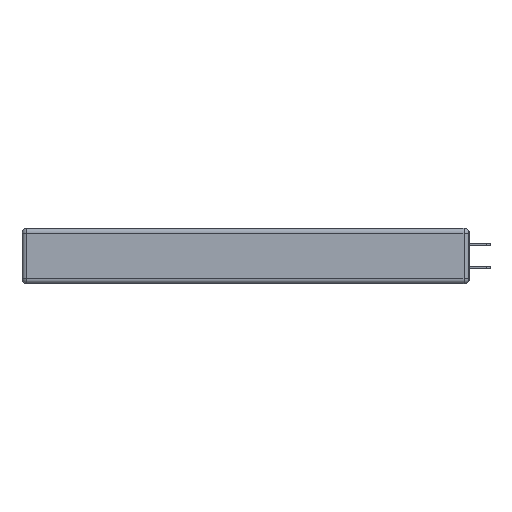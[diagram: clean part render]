
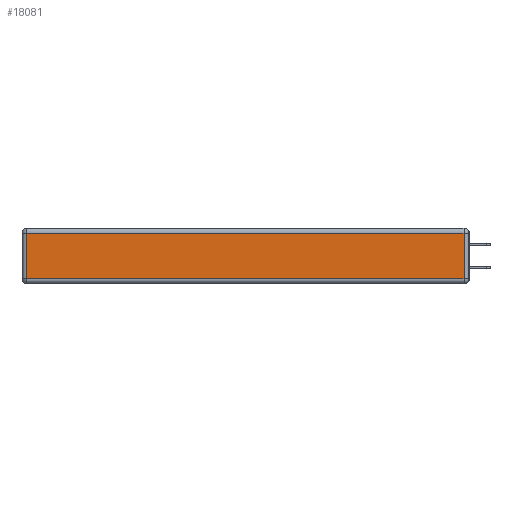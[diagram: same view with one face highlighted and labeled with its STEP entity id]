
A CAD part, left-side view. The second image highlights one B-rep face of the part: STEP entity #18081.
In plain terms, the highlighted planar face has unit normal (-1, 0, 0).
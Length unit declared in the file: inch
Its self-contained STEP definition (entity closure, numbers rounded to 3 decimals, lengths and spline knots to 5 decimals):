
#25 = VECTOR ( 'NONE', #11373, 39.37008 ) ;
#868 = DIRECTION ( 'NONE',  ( 0., 0., 1. ) ) ;
#2561 = VECTOR ( 'NONE', #9159, 39.37008 ) ;
#3743 = LINE ( 'NONE', #17211, #8908 ) ;
#4259 = ORIENTED_EDGE ( 'NONE', *, *, #6873, .T. ) ;
#4557 = CARTESIAN_POINT ( 'NONE',  ( 0., 0.03, -0.313 ) ) ;
#4997 = CARTESIAN_POINT ( 'NONE',  ( 0., 2.72, -0.03 ) ) ;
#5650 = LINE ( 'NONE', #8458, #14462 ) ;
#6099 = CARTESIAN_POINT ( 'NONE',  ( 0., 0., -0.343 ) ) ;
#6133 = EDGE_LOOP ( 'NONE', ( #9773, #18036, #4259, #8111 ) ) ;
#6395 = FACE_OUTER_BOUND ( 'NONE', #6133, .T. ) ;
#6404 = DIRECTION ( 'NONE',  ( 0., 0., -1. ) ) ;
#6873 = EDGE_CURVE ( 'NONE', #15932, #14749, #8455, .T. ) ;
#7755 = DIRECTION ( 'NONE',  ( 0., 0., 1. ) ) ;
#8111 = ORIENTED_EDGE ( 'NONE', *, *, #8340, .T. ) ;
#8228 = VERTEX_POINT ( 'NONE', #4557 ) ;
#8340 = EDGE_CURVE ( 'NONE', #14749, #11063, #3743, .T. ) ;
#8455 = LINE ( 'NONE', #9088, #2561 ) ;
#8458 = CARTESIAN_POINT ( 'NONE',  ( 0., 0.03, -0.343 ) ) ;
#8908 = VECTOR ( 'NONE', #6404, 39.37008 ) ;
#9088 = CARTESIAN_POINT ( 'NONE',  ( 0., 2.75, -0.03 ) ) ;
#9159 = DIRECTION ( 'NONE',  ( 0., 1., 0. ) ) ;
#9482 = CARTESIAN_POINT ( 'NONE',  ( 0., 0.03, -0.03 ) ) ;
#9773 = ORIENTED_EDGE ( 'NONE', *, *, #18363, .T. ) ;
#10774 = LINE ( 'NONE', #19182, #25 ) ;
#11063 = VERTEX_POINT ( 'NONE', #19878 ) ;
#11373 = DIRECTION ( 'NONE',  ( 0., -1., 0. ) ) ;
#13700 = PLANE ( 'NONE',  #15072 ) ;
#14462 = VECTOR ( 'NONE', #868, 39.37008 ) ;
#14749 = VERTEX_POINT ( 'NONE', #4997 ) ;
#15072 = AXIS2_PLACEMENT_3D ( 'NONE', #6099, #18634, #7755 ) ;
#15932 = VERTEX_POINT ( 'NONE', #9482 ) ;
#17211 = CARTESIAN_POINT ( 'NONE',  ( 0., 2.72, -0.343 ) ) ;
#17861 = EDGE_CURVE ( 'NONE', #8228, #15932, #5650, .T. ) ;
#18036 = ORIENTED_EDGE ( 'NONE', *, *, #17861, .T. ) ;
#18081 = ADVANCED_FACE ( 'NONE', ( #6395 ), #13700, .T. ) ;
#18363 = EDGE_CURVE ( 'NONE', #11063, #8228, #10774, .T. ) ;
#18634 = DIRECTION ( 'NONE',  ( -1., 0., 0. ) ) ;
#19182 = CARTESIAN_POINT ( 'NONE',  ( 0., 0., -0.313 ) ) ;
#19878 = CARTESIAN_POINT ( 'NONE',  ( 0., 2.72, -0.313 ) ) ;
